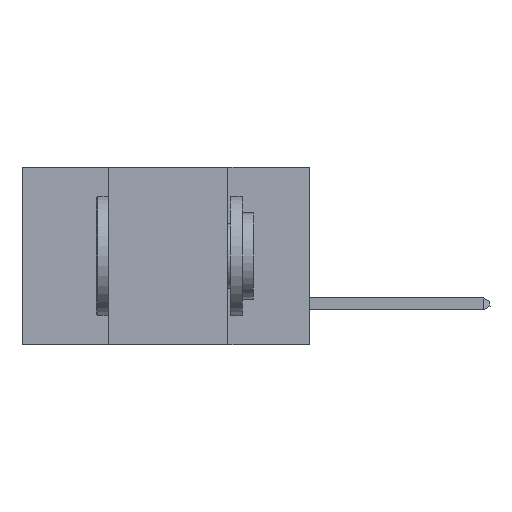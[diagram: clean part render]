
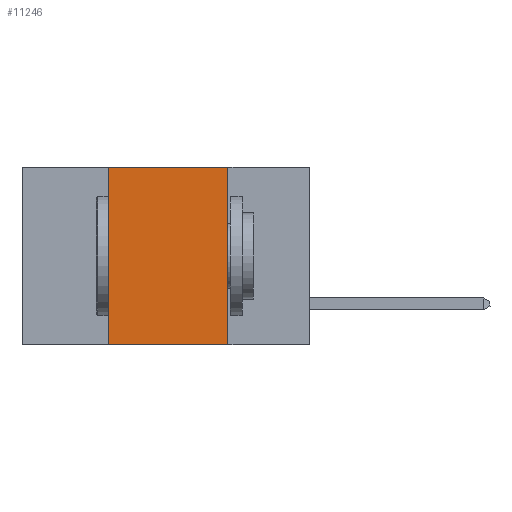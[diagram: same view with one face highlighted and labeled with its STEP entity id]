
A CAD part, left-side view. The second image highlights one B-rep face of the part: STEP entity #11246.
In plain terms, the highlighted planar face has unit normal (-1, 0, 0).
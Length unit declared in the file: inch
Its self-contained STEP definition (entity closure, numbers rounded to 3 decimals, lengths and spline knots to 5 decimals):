
#392 = CARTESIAN_POINT ( 'NONE',  ( 0., 0.42, 0. ) ) ;
#911 = CARTESIAN_POINT ( 'NONE',  ( 0., 0.6, -0.37 ) ) ;
#941 = LINE ( 'NONE', #392, #1364 ) ;
#1364 = VECTOR ( 'NONE', #11514, 39.37008 ) ;
#1931 = CARTESIAN_POINT ( 'NONE',  ( 0., 0.42, 0. ) ) ;
#2028 = LINE ( 'NONE', #15299, #6865 ) ;
#2037 = ORIENTED_EDGE ( 'NONE', *, *, #2783, .F. ) ;
#2230 = VERTEX_POINT ( 'NONE', #16696 ) ;
#2614 = CARTESIAN_POINT ( 'NONE',  ( 0., 0.17, -0.37 ) ) ;
#2783 = EDGE_CURVE ( 'NONE', #2230, #4387, #12642, .T. ) ;
#2785 = CARTESIAN_POINT ( 'NONE',  ( 0., 0.6, 0. ) ) ;
#2847 = DIRECTION ( 'NONE',  ( 0., 0., -1. ) ) ;
#3423 = ORIENTED_EDGE ( 'NONE', *, *, #16695, .F. ) ;
#4387 = VERTEX_POINT ( 'NONE', #2614 ) ;
#4449 = LINE ( 'NONE', #911, #15048 ) ;
#4667 = VERTEX_POINT ( 'NONE', #1931 ) ;
#5029 = DIRECTION ( 'NONE',  ( 0., 0., -1. ) ) ;
#5152 = AXIS2_PLACEMENT_3D ( 'NONE', #2785, #10842, #2847 ) ;
#5335 = EDGE_CURVE ( 'NONE', #11010, #4387, #4449, .T. ) ;
#6865 = VECTOR ( 'NONE', #7303, 39.37008 ) ;
#7303 = DIRECTION ( 'NONE',  ( 0., -1., 0. ) ) ;
#8882 = EDGE_CURVE ( 'NONE', #11010, #4667, #941, .T. ) ;
#9604 = PLANE ( 'NONE',  #5152 ) ;
#9646 = EDGE_LOOP ( 'NONE', ( #2037, #3423, #12176, #12818 ) ) ;
#9880 = VECTOR ( 'NONE', #5029, 39.37008 ) ;
#10842 = DIRECTION ( 'NONE',  ( 1., 0., 0. ) ) ;
#11010 = VERTEX_POINT ( 'NONE', #17066 ) ;
#11246 = ADVANCED_FACE ( 'NONE', ( #15370 ), #9604, .F. ) ;
#11514 = DIRECTION ( 'NONE',  ( 0., 0., 1. ) ) ;
#12176 = ORIENTED_EDGE ( 'NONE', *, *, #8882, .F. ) ;
#12642 = LINE ( 'NONE', #14442, #9880 ) ;
#12818 = ORIENTED_EDGE ( 'NONE', *, *, #5335, .T. ) ;
#14442 = CARTESIAN_POINT ( 'NONE',  ( 0., 0.17, 0. ) ) ;
#15048 = VECTOR ( 'NONE', #17265, 39.37008 ) ;
#15299 = CARTESIAN_POINT ( 'NONE',  ( 0., 0.6, 0. ) ) ;
#15370 = FACE_OUTER_BOUND ( 'NONE', #9646, .T. ) ;
#16695 = EDGE_CURVE ( 'NONE', #4667, #2230, #2028, .T. ) ;
#16696 = CARTESIAN_POINT ( 'NONE',  ( 0., 0.17, 0. ) ) ;
#17066 = CARTESIAN_POINT ( 'NONE',  ( 0., 0.42, -0.37 ) ) ;
#17265 = DIRECTION ( 'NONE',  ( 0., -1., 0. ) ) ;
